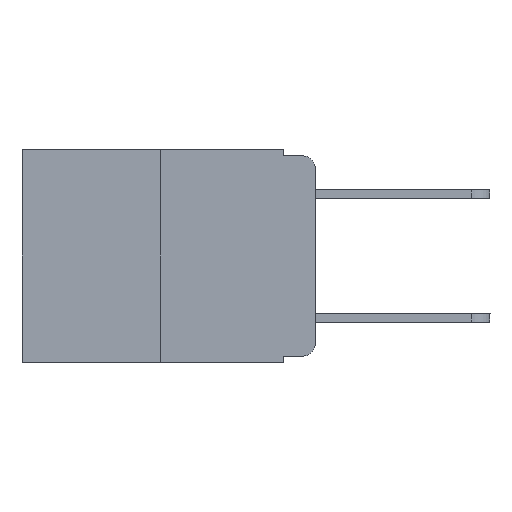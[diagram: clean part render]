
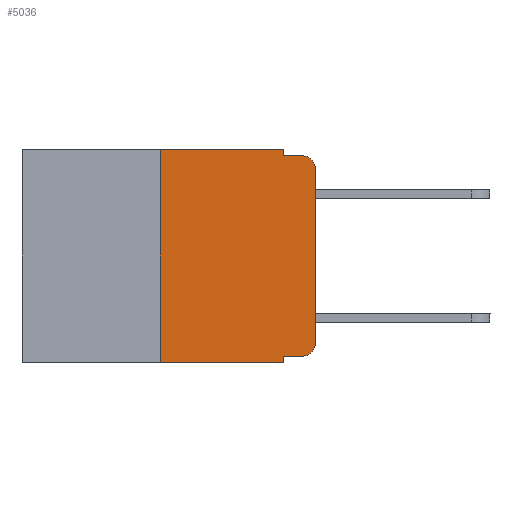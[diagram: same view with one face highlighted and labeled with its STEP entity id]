
A CAD part, left-side view. The second image highlights one B-rep face of the part: STEP entity #5036.
In plain terms, the highlighted planar face has unit normal (-1, 0, 0).
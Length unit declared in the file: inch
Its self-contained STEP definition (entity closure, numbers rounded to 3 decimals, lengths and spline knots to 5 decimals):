
#40 = CARTESIAN_POINT ( 'NONE',  ( 0., 0.051, -0.343 ) ) ;
#175 = VECTOR ( 'NONE', #4155, 39.37008 ) ;
#335 = DIRECTION ( 'NONE',  ( 0., 0., -1. ) ) ;
#489 = CARTESIAN_POINT ( 'NONE',  ( 0., 0.473, -0.343 ) ) ;
#616 = CARTESIAN_POINT ( 'NONE',  ( 0., 0.25, -0.343 ) ) ;
#699 = EDGE_CURVE ( 'NONE', #10553, #1256, #8306, .T. ) ;
#846 = AXIS2_PLACEMENT_3D ( 'NONE', #7086, #10131, #8158 ) ;
#922 = CARTESIAN_POINT ( 'NONE',  ( 0., 0.051, -0.01 ) ) ;
#930 = VECTOR ( 'NONE', #11186, 39.37008 ) ;
#944 = CIRCLE ( 'NONE', #11466, 0.02 ) ;
#1090 = VERTEX_POINT ( 'NONE', #7751 ) ;
#1095 = EDGE_CURVE ( 'NONE', #8560, #4694, #944, .T. ) ;
#1254 = EDGE_CURVE ( 'NONE', #9882, #3092, #3968, .T. ) ;
#1256 = VERTEX_POINT ( 'NONE', #40 ) ;
#1396 = CARTESIAN_POINT ( 'NONE',  ( 0., 0.02, -0.313 ) ) ;
#1447 = LINE ( 'NONE', #9648, #3351 ) ;
#1911 = LINE ( 'NONE', #12622, #7034 ) ;
#1971 = EDGE_CURVE ( 'NONE', #3092, #4552, #9986, .T. ) ;
#2056 = ORIENTED_EDGE ( 'NONE', *, *, #10411, .T. ) ;
#2058 = EDGE_CURVE ( 'NONE', #1090, #13151, #7153, .T. ) ;
#3046 = CARTESIAN_POINT ( 'NONE',  ( 0., 0.25, 0. ) ) ;
#3092 = VERTEX_POINT ( 'NONE', #3046 ) ;
#3201 = CARTESIAN_POINT ( 'NONE',  ( 0., 0.051, -0.01 ) ) ;
#3351 = VECTOR ( 'NONE', #12703, 39.37008 ) ;
#3390 = LINE ( 'NONE', #489, #4357 ) ;
#3608 = ORIENTED_EDGE ( 'NONE', *, *, #9990, .T. ) ;
#3968 = LINE ( 'NONE', #12261, #930 ) ;
#3988 = ORIENTED_EDGE ( 'NONE', *, *, #9244, .F. ) ;
#4042 = EDGE_CURVE ( 'NONE', #10553, #8560, #1447, .T. ) ;
#4155 = DIRECTION ( 'NONE',  ( 0., 0., 1. ) ) ;
#4357 = VECTOR ( 'NONE', #7646, 39.37008 ) ;
#4552 = VERTEX_POINT ( 'NONE', #10386 ) ;
#4694 = VERTEX_POINT ( 'NONE', #7557 ) ;
#4712 = ORIENTED_EDGE ( 'NONE', *, *, #2058, .T. ) ;
#4899 = CARTESIAN_POINT ( 'NONE',  ( 0., 0.02, -0.333 ) ) ;
#5036 = ADVANCED_FACE ( 'NONE', ( #10185 ), #9062, .F. ) ;
#5358 = CARTESIAN_POINT ( 'NONE',  ( 0., 0.02, -0.03 ) ) ;
#5521 = ORIENTED_EDGE ( 'NONE', *, *, #4042, .T. ) ;
#5881 = AXIS2_PLACEMENT_3D ( 'NONE', #5358, #11528, #335 ) ;
#6276 = ORIENTED_EDGE ( 'NONE', *, *, #1095, .T. ) ;
#6388 = DIRECTION ( 'NONE',  ( 0., -1., 0. ) ) ;
#6524 = CARTESIAN_POINT ( 'NONE',  ( 0., 0.02, -0.01 ) ) ;
#6968 = DIRECTION ( 'NONE',  ( 0., -1., 0. ) ) ;
#7034 = VECTOR ( 'NONE', #12797, 39.37008 ) ;
#7045 = CARTESIAN_POINT ( 'NONE',  ( 0., 0.051, 0. ) ) ;
#7086 = CARTESIAN_POINT ( 'NONE',  ( 0., 0.473, 0. ) ) ;
#7153 = CIRCLE ( 'NONE', #5881, 0.02 ) ;
#7244 = CARTESIAN_POINT ( 'NONE',  ( 0., 0., 0. ) ) ;
#7418 = CARTESIAN_POINT ( 'NONE',  ( 0., 0.051, -0.333 ) ) ;
#7557 = CARTESIAN_POINT ( 'NONE',  ( 0., 0., -0.313 ) ) ;
#7646 = DIRECTION ( 'NONE',  ( 0., -1., 0. ) ) ;
#7751 = CARTESIAN_POINT ( 'NONE',  ( 0., 0., -0.03 ) ) ;
#7812 = ORIENTED_EDGE ( 'NONE', *, *, #699, .F. ) ;
#8158 = DIRECTION ( 'NONE',  ( 0., 0., -1. ) ) ;
#8201 = DIRECTION ( 'NONE',  ( 0., 0., -1. ) ) ;
#8306 = LINE ( 'NONE', #7045, #12428 ) ;
#8313 = CARTESIAN_POINT ( 'NONE',  ( 0., 0.473, 0. ) ) ;
#8560 = VERTEX_POINT ( 'NONE', #4899 ) ;
#8841 = VERTEX_POINT ( 'NONE', #3201 ) ;
#9062 = PLANE ( 'NONE',  #846 ) ;
#9244 = EDGE_CURVE ( 'NONE', #8841, #13151, #9419, .T. ) ;
#9419 = LINE ( 'NONE', #922, #11809 ) ;
#9648 = CARTESIAN_POINT ( 'NONE',  ( 0., 0.051, -0.333 ) ) ;
#9832 = VECTOR ( 'NONE', #6388, 39.37008 ) ;
#9882 = VERTEX_POINT ( 'NONE', #616 ) ;
#9986 = LINE ( 'NONE', #8313, #9832 ) ;
#9990 = EDGE_CURVE ( 'NONE', #9882, #1256, #3390, .T. ) ;
#10131 = DIRECTION ( 'NONE',  ( 1., 0., 0. ) ) ;
#10185 = FACE_OUTER_BOUND ( 'NONE', #12271, .T. ) ;
#10211 = ORIENTED_EDGE ( 'NONE', *, *, #1971, .F. ) ;
#10386 = CARTESIAN_POINT ( 'NONE',  ( 0., 0.051, 0. ) ) ;
#10411 = EDGE_CURVE ( 'NONE', #4694, #1090, #10716, .T. ) ;
#10553 = VERTEX_POINT ( 'NONE', #7418 ) ;
#10716 = LINE ( 'NONE', #7244, #175 ) ;
#11186 = DIRECTION ( 'NONE',  ( 0., 0., 1. ) ) ;
#11466 = AXIS2_PLACEMENT_3D ( 'NONE', #1396, #11759, #12824 ) ;
#11528 = DIRECTION ( 'NONE',  ( -1., 0., 0. ) ) ;
#11759 = DIRECTION ( 'NONE',  ( -1., 0., 0. ) ) ;
#11789 = ORIENTED_EDGE ( 'NONE', *, *, #12112, .F. ) ;
#11809 = VECTOR ( 'NONE', #6968, 39.37008 ) ;
#12112 = EDGE_CURVE ( 'NONE', #4552, #8841, #1911, .T. ) ;
#12261 = CARTESIAN_POINT ( 'NONE',  ( 0., 0.25, 0. ) ) ;
#12271 = EDGE_LOOP ( 'NONE', ( #2056, #4712, #3988, #11789, #10211, #13045, #3608, #7812, #5521, #6276 ) ) ;
#12428 = VECTOR ( 'NONE', #8201, 39.37008 ) ;
#12622 = CARTESIAN_POINT ( 'NONE',  ( 0., 0.051, 0. ) ) ;
#12703 = DIRECTION ( 'NONE',  ( 0., -1., 0. ) ) ;
#12797 = DIRECTION ( 'NONE',  ( 0., 0., -1. ) ) ;
#12824 = DIRECTION ( 'NONE',  ( 0., 0., -1. ) ) ;
#13045 = ORIENTED_EDGE ( 'NONE', *, *, #1254, .F. ) ;
#13151 = VERTEX_POINT ( 'NONE', #6524 ) ;
